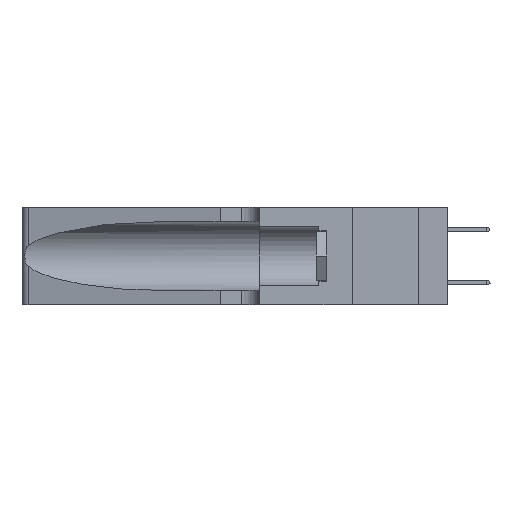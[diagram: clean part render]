
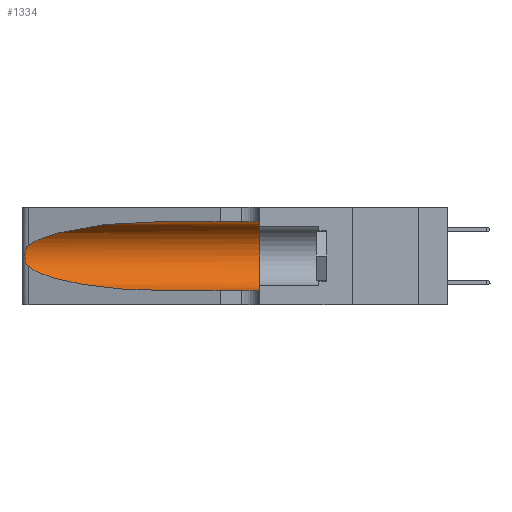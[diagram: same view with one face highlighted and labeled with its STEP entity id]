
A CAD part, left-side view. The second image highlights one B-rep face of the part: STEP entity #1334.
In plain terms, the highlighted cylindrical face has radius 3.308 mm (diameter 6.617 mm), a partial arc.
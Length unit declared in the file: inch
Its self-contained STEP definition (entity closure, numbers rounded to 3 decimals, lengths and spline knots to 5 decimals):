
#33 = VERTEX_POINT ( 'NONE', #10368 ) ;
#387 = EDGE_CURVE ( 'NONE', #19693, #9428, #1171, .T. ) ;
#435 =( BOUNDED_CURVE ( )  B_SPLINE_CURVE ( 3, ( #20460, #11587, #18747, #8137 ),
 .UNSPECIFIED., .F., .F. ) 
 B_SPLINE_CURVE_WITH_KNOTS ( ( 4, 4 ),
 ( 3.44316, 4.71239 ),
 .UNSPECIFIED. ) 
 CURVE ( )  GEOMETRIC_REPRESENTATION_ITEM ( )  RATIONAL_B_SPLINE_CURVE ( ( 1., 0.87, 0.87, 1. ) ) 
 REPRESENTATION_ITEM ( '' )  );
#877 = ORIENTED_EDGE ( 'NONE', *, *, #16051, .T. ) ;
#1171 =( BOUNDED_CURVE ( )  B_SPLINE_CURVE ( 3, ( #3276, #19151, #17534, #12298 ),
 .UNSPECIFIED., .F., .T. ) 
 B_SPLINE_CURVE_WITH_KNOTS ( ( 4, 4 ),
 ( 1.5708, 2.84003 ),
 .UNSPECIFIED. ) 
 CURVE ( )  GEOMETRIC_REPRESENTATION_ITEM ( )  RATIONAL_B_SPLINE_CURVE ( ( 1., 0.87, 0.87, 1. ) ) 
 REPRESENTATION_ITEM ( '' )  );
#1319 = CARTESIAN_POINT ( 'NONE',  ( 0.25639, 1.23184, 0.21858 ) ) ;
#1334 = ADVANCED_FACE ( 'NONE', ( #11413 ), #14506, .F. ) ;
#1711 = ORIENTED_EDGE ( 'NONE', *, *, #2987, .T. ) ;
#1785 = CARTESIAN_POINT ( 'NONE',  ( 0.25487, 1.22718, 0.22369 ) ) ;
#1979 = CARTESIAN_POINT ( 'NONE',  ( 0.1305, 0.72297, 0.31525 ) ) ;
#2097 = ORIENTED_EDGE ( 'NONE', *, *, #6972, .F. ) ;
#2987 = EDGE_CURVE ( 'NONE', #9428, #8929, #16272, .T. ) ;
#3274 = CARTESIAN_POINT ( 'NONE',  ( 0.26018, 1.23835, 0.19895 ) ) ;
#3276 = CARTESIAN_POINT ( 'NONE',  ( 0.1305, 0.72297, 0.31525 ) ) ;
#4613 = AXIS2_PLACEMENT_3D ( 'NONE', #17429, #8509, #17290 ) ;
#4975 = CARTESIAN_POINT ( 'NONE',  ( 0.25487, 1.22718, 0.22369 ) ) ;
#5008 = CARTESIAN_POINT ( 'NONE',  ( 0.1305, 1.61858, 0.185 ) ) ;
#5131 = CARTESIAN_POINT ( 'NONE',  ( 0.25789, 1.23486, 0.15765 ) ) ;
#5879 = VECTOR ( 'NONE', #7248, 39.37008 ) ;
#6003 = CARTESIAN_POINT ( 'NONE',  ( 0.1305, 1.61858, 0.05475 ) ) ;
#6302 = ORIENTED_EDGE ( 'NONE', *, *, #387, .T. ) ;
#6772 = CARTESIAN_POINT ( 'NONE',  ( 0.25555, 1.22994, 0.2215 ) ) ;
#6972 = EDGE_CURVE ( 'NONE', #19693, #8180, #6991, .T. ) ;
#6991 = LINE ( 'NONE', #10614, #5879 ) ;
#7248 = DIRECTION ( 'NONE',  ( 0., -1., 0. ) ) ;
#7470 = EDGE_CURVE ( 'NONE', #8180, #15353, #13314, .T. ) ;
#7547 = DIRECTION ( 'NONE',  ( 0., -1., 0. ) ) ;
#7928 = CARTESIAN_POINT ( 'NONE',  ( 0.1305, 0.35, 0.31525 ) ) ;
#8137 = CARTESIAN_POINT ( 'NONE',  ( 0.1305, 0.72297, 0.05475 ) ) ;
#8180 = VERTEX_POINT ( 'NONE', #7928 ) ;
#8509 = DIRECTION ( 'NONE',  ( 0., 1., 0. ) ) ;
#8929 = VERTEX_POINT ( 'NONE', #17683 ) ;
#9428 = VERTEX_POINT ( 'NONE', #1785 ) ;
#10360 = CARTESIAN_POINT ( 'NONE',  ( 0.26075, 1.23896, 0.178 ) ) ;
#10368 = CARTESIAN_POINT ( 'NONE',  ( 0.1305, 0.72297, 0.05475 ) ) ;
#10614 = CARTESIAN_POINT ( 'NONE',  ( 0.1305, 1.61858, 0.31525 ) ) ;
#11253 = EDGE_LOOP ( 'NONE', ( #6302, #1711, #877, #22033, #21606, #2097 ) ) ;
#11413 = FACE_OUTER_BOUND ( 'NONE', #11253, .T. ) ;
#11587 = CARTESIAN_POINT ( 'NONE',  ( 0.2373, 1.15595, 0.08982 ) ) ;
#12143 = CARTESIAN_POINT ( 'NONE',  ( 0.25856, 1.23593, 0.16098 ) ) ;
#12298 = CARTESIAN_POINT ( 'NONE',  ( 0.25487, 1.22718, 0.22369 ) ) ;
#12942 = CARTESIAN_POINT ( 'NONE',  ( 0.1305, 0.35, 0.05475 ) ) ;
#13240 = VECTOR ( 'NONE', #7547, 39.37008 ) ;
#13314 = CIRCLE ( 'NONE', #4613, 0.13025 ) ;
#13870 = CARTESIAN_POINT ( 'NONE',  ( 0.25854, 1.2359, 0.20912 ) ) ;
#14341 = CARTESIAN_POINT ( 'NONE',  ( 0.25487, 1.22718, 0.14631 ) ) ;
#14506 = CYLINDRICAL_SURFACE ( 'NONE', #19233, 0.13025 ) ;
#15353 = VERTEX_POINT ( 'NONE', #12942 ) ;
#15568 = EDGE_CURVE ( 'NONE', #33, #15353, #19099, .T. ) ;
#15698 = CARTESIAN_POINT ( 'NONE',  ( 0.26075, 1.23896, 0.19203 ) ) ;
#16051 = EDGE_CURVE ( 'NONE', #8929, #33, #435, .T. ) ;
#16222 = CARTESIAN_POINT ( 'NONE',  ( 0.25555, 1.22993, 0.14849 ) ) ;
#16272 = B_SPLINE_CURVE_WITH_KNOTS ( 'NONE', 3,
 ( #4975, #6772, #1319, #19150, #13870, #3274, #15698, #10360, #22792, #12143, #5131, #17532, #16222, #14341 ),
 .UNSPECIFIED., .F., .F.,
 ( 4, 2, 2, 2, 2, 2, 4 ),
 ( 0., 0.00027, 0.00053, 0.00107, 0.0016, 0.00187, 0.00214 ),
 .UNSPECIFIED. ) ;
#17290 = DIRECTION ( 'NONE',  ( 0., 0., 1. ) ) ;
#17423 = DIRECTION ( 'NONE',  ( 0., -1., 0. ) ) ;
#17429 = CARTESIAN_POINT ( 'NONE',  ( 0.1305, 0.35, 0.185 ) ) ;
#17532 = CARTESIAN_POINT ( 'NONE',  ( 0.25639, 1.23186, 0.15144 ) ) ;
#17534 = CARTESIAN_POINT ( 'NONE',  ( 0.2373, 1.15595, 0.28018 ) ) ;
#17683 = CARTESIAN_POINT ( 'NONE',  ( 0.25487, 1.22718, 0.14631 ) ) ;
#18747 = CARTESIAN_POINT ( 'NONE',  ( 0.18966, 0.96281, 0.05475 ) ) ;
#19099 = LINE ( 'NONE', #6003, #13240 ) ;
#19150 = CARTESIAN_POINT ( 'NONE',  ( 0.25787, 1.23484, 0.2124 ) ) ;
#19151 = CARTESIAN_POINT ( 'NONE',  ( 0.18966, 0.96281, 0.31525 ) ) ;
#19233 = AXIS2_PLACEMENT_3D ( 'NONE', #5008, #17423, #19411 ) ;
#19411 = DIRECTION ( 'NONE',  ( 0., 0., -1. ) ) ;
#19693 = VERTEX_POINT ( 'NONE', #1979 ) ;
#20460 = CARTESIAN_POINT ( 'NONE',  ( 0.25487, 1.22718, 0.14631 ) ) ;
#21606 = ORIENTED_EDGE ( 'NONE', *, *, #7470, .F. ) ;
#22033 = ORIENTED_EDGE ( 'NONE', *, *, #15568, .T. ) ;
#22792 = CARTESIAN_POINT ( 'NONE',  ( 0.26017, 1.23833, 0.17102 ) ) ;
